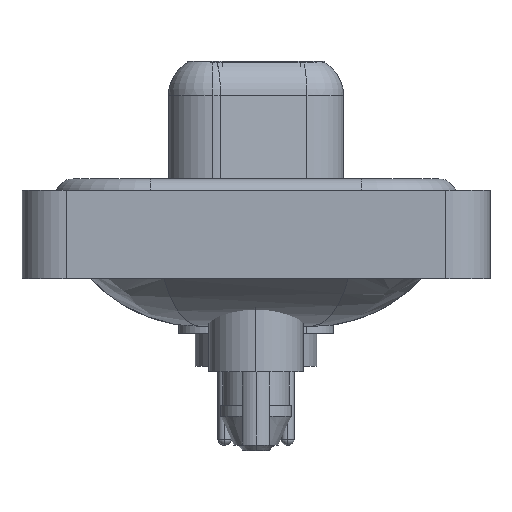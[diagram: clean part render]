
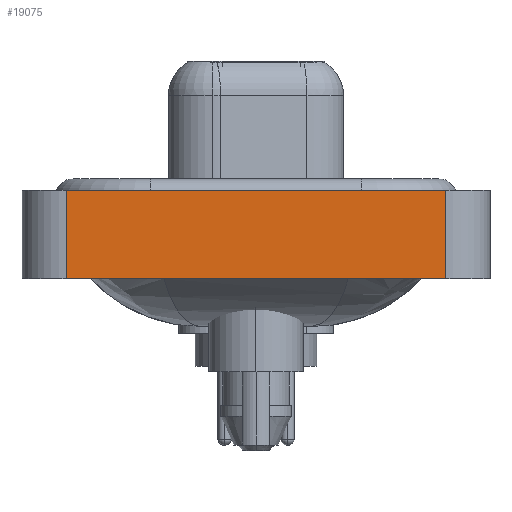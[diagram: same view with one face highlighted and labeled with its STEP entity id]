
A CAD part, left-side view. The second image highlights one B-rep face of the part: STEP entity #19075.
In plain terms, the highlighted planar face has unit normal (-1, 0, 0).
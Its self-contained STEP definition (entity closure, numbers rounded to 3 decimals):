
#339 = VERTEX_POINT ( 'NONE', #2280 ) ;
#1087 = DIRECTION ( 'NONE',  ( 0., -1., 0. ) ) ;
#2097 = LINE ( 'NONE', #10120, #3868 ) ;
#2280 = CARTESIAN_POINT ( 'NONE',  ( -7.35, 8.55, 0.4 ) ) ;
#2601 = VERTEX_POINT ( 'NONE', #11290 ) ;
#2681 = VECTOR ( 'NONE', #1087, 1000. ) ;
#2923 = LINE ( 'NONE', #25254, #2681 ) ;
#3140 = CARTESIAN_POINT ( 'NONE',  ( -7.35, 8.55, -3.6 ) ) ;
#3868 = VECTOR ( 'NONE', #4479, 1000. ) ;
#4479 = DIRECTION ( 'NONE',  ( 0., 0., 1. ) ) ;
#5615 = EDGE_LOOP ( 'NONE', ( #15437, #14299, #16641, #6013 ) ) ;
#5848 = CARTESIAN_POINT ( 'NONE',  ( -7.35, -8.55, -3.6 ) ) ;
#6013 = ORIENTED_EDGE ( 'NONE', *, *, #7218, .T. ) ;
#7218 = EDGE_CURVE ( 'NONE', #9287, #18270, #10277, .T. ) ;
#7696 = PLANE ( 'NONE',  #22372 ) ;
#9061 = EDGE_CURVE ( 'NONE', #18270, #2601, #2097, .T. ) ;
#9287 = VERTEX_POINT ( 'NONE', #11554 ) ;
#10120 = CARTESIAN_POINT ( 'NONE',  ( -7.35, -8.55, -3.6 ) ) ;
#10277 = LINE ( 'NONE', #14356, #25179 ) ;
#10778 = LINE ( 'NONE', #3140, #21663 ) ;
#11290 = CARTESIAN_POINT ( 'NONE',  ( -7.35, -8.55, 0.4 ) ) ;
#11554 = CARTESIAN_POINT ( 'NONE',  ( -7.35, 8.55, -3.6 ) ) ;
#11780 = DIRECTION ( 'NONE',  ( -1., 0., 0. ) ) ;
#12649 = DIRECTION ( 'NONE',  ( 0., -1., 0. ) ) ;
#14299 = ORIENTED_EDGE ( 'NONE', *, *, #19647, .F. ) ;
#14356 = CARTESIAN_POINT ( 'NONE',  ( -7.35, -8.55, -3.6 ) ) ;
#14853 = DIRECTION ( 'NONE',  ( 0., 0., 1. ) ) ;
#15437 = ORIENTED_EDGE ( 'NONE', *, *, #9061, .T. ) ;
#16641 = ORIENTED_EDGE ( 'NONE', *, *, #18119, .F. ) ;
#17680 = FACE_OUTER_BOUND ( 'NONE', #5615, .T. ) ;
#18119 = EDGE_CURVE ( 'NONE', #9287, #339, #10778, .T. ) ;
#18270 = VERTEX_POINT ( 'NONE', #5848 ) ;
#19075 = ADVANCED_FACE ( 'NONE', ( #17680 ), #7696, .T. ) ;
#19647 = EDGE_CURVE ( 'NONE', #339, #2601, #2923, .T. ) ;
#19774 = DIRECTION ( 'NONE',  ( 0., 0., 1. ) ) ;
#21663 = VECTOR ( 'NONE', #14853, 1000. ) ;
#22372 = AXIS2_PLACEMENT_3D ( 'NONE', #25708, #11780, #19774 ) ;
#25179 = VECTOR ( 'NONE', #12649, 1000. ) ;
#25254 = CARTESIAN_POINT ( 'NONE',  ( -7.35, -8.55, 0.4 ) ) ;
#25708 = CARTESIAN_POINT ( 'NONE',  ( -7.35, -8.55, -3.6 ) ) ;
